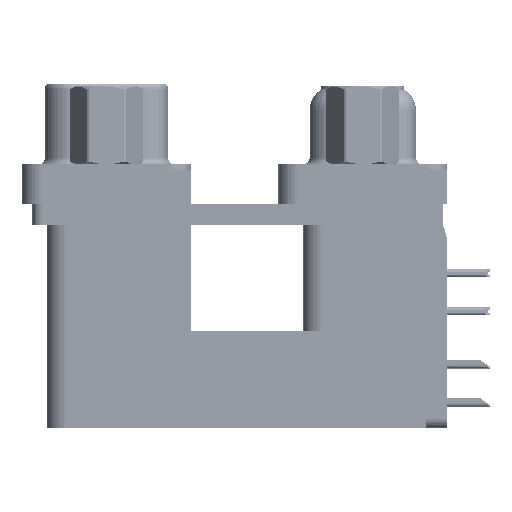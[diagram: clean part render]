
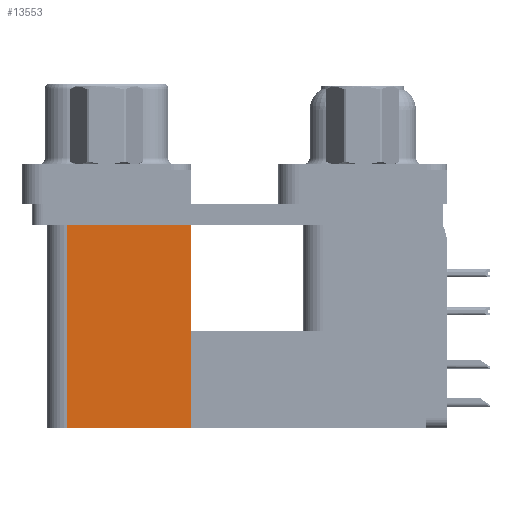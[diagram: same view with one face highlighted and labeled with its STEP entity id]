
A CAD part, left-side view. The second image highlights one B-rep face of the part: STEP entity #13553.
In plain terms, the highlighted planar face has unit normal (-1, 0, 0).
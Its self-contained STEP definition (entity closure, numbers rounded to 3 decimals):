
#341 = CARTESIAN_POINT ( 'NONE',  ( 3.79, 21.975, -19.2 ) ) ;
#525 = DIRECTION ( 'NONE',  ( 1., 0., 0. ) ) ;
#862 = CARTESIAN_POINT ( 'NONE',  ( 3.79, 12.775, -19.2 ) ) ;
#1825 = LINE ( 'NONE', #24187, #27073 ) ;
#3749 = LINE ( 'NONE', #67755, #69370 ) ;
#5869 = LINE ( 'NONE', #71662, #67019 ) ;
#6661 = VERTEX_POINT ( 'NONE', #341 ) ;
#6720 = DIRECTION ( 'NONE',  ( 0., 1., 0. ) ) ;
#9689 = DIRECTION ( 'NONE',  ( 0., 1., 0. ) ) ;
#11516 = ORIENTED_EDGE ( 'NONE', *, *, #66395, .T. ) ;
#12019 = VERTEX_POINT ( 'NONE', #20692 ) ;
#13553 = ADVANCED_FACE ( 'NONE', ( #34944 ), #62825, .F. ) ;
#20181 = CARTESIAN_POINT ( 'NONE',  ( 3.79, 12.775, -2.5 ) ) ;
#20692 = CARTESIAN_POINT ( 'NONE',  ( 3.79, 12.775, -19.2 ) ) ;
#21251 = AXIS2_PLACEMENT_3D ( 'NONE', #862, #525, #6720 ) ;
#24187 = CARTESIAN_POINT ( 'NONE',  ( 3.79, 12.775, -19.2 ) ) ;
#25161 = ORIENTED_EDGE ( 'NONE', *, *, #63074, .F. ) ;
#27073 = VECTOR ( 'NONE', #68562, 1000. ) ;
#32821 = EDGE_CURVE ( 'NONE', #12019, #6661, #3749, .T. ) ;
#34944 = FACE_OUTER_BOUND ( 'NONE', #50947, .T. ) ;
#36784 = LINE ( 'NONE', #59153, #37266 ) ;
#37127 = DIRECTION ( 'NONE',  ( 0., 0., 1. ) ) ;
#37266 = VECTOR ( 'NONE', #37127, 1000. ) ;
#37464 = VERTEX_POINT ( 'NONE', #46071 ) ;
#42955 = DIRECTION ( 'NONE',  ( 0., 1., 0. ) ) ;
#46071 = CARTESIAN_POINT ( 'NONE',  ( 3.79, 21.975, -2.5 ) ) ;
#50947 = EDGE_LOOP ( 'NONE', ( #72486, #25161, #58558, #11516 ) ) ;
#54093 = VERTEX_POINT ( 'NONE', #20181 ) ;
#58558 = ORIENTED_EDGE ( 'NONE', *, *, #32821, .F. ) ;
#59153 = CARTESIAN_POINT ( 'NONE',  ( 3.79, 21.975, -19.2 ) ) ;
#62825 = PLANE ( 'NONE',  #21251 ) ;
#63074 = EDGE_CURVE ( 'NONE', #6661, #37464, #36784, .T. ) ;
#66395 = EDGE_CURVE ( 'NONE', #12019, #54093, #1825, .T. ) ;
#67019 = VECTOR ( 'NONE', #9689, 1000. ) ;
#67285 = EDGE_CURVE ( 'NONE', #54093, #37464, #5869, .T. ) ;
#67755 = CARTESIAN_POINT ( 'NONE',  ( 3.79, 12.775, -19.2 ) ) ;
#68562 = DIRECTION ( 'NONE',  ( 0., 0., 1. ) ) ;
#69370 = VECTOR ( 'NONE', #42955, 1000. ) ;
#71662 = CARTESIAN_POINT ( 'NONE',  ( 3.79, 12.775, -2.5 ) ) ;
#72486 = ORIENTED_EDGE ( 'NONE', *, *, #67285, .T. ) ;
